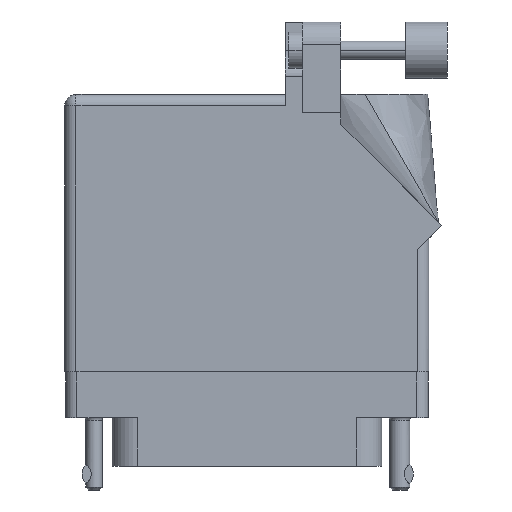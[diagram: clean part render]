
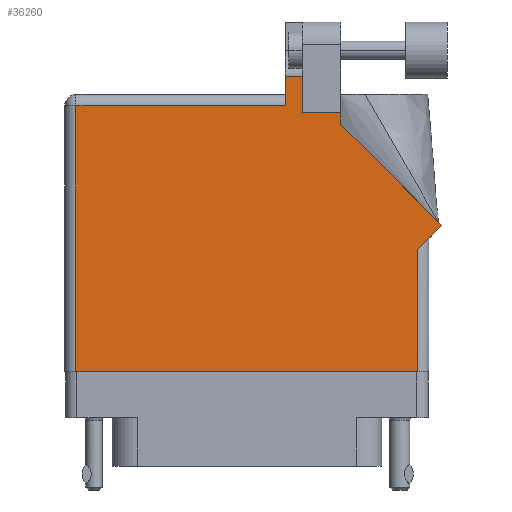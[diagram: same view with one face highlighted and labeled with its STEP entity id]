
A CAD part, front view. The second image highlights one B-rep face of the part: STEP entity #36260.
In plain terms, the highlighted face is planar.
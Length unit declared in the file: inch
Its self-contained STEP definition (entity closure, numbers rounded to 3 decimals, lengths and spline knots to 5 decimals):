
#535 = LINE ( 'NONE', #37012, #33537 ) ;
#968 = DIRECTION ( 'NONE',  ( -1., 0., 0. ) ) ;
#1126 = CARTESIAN_POINT ( 'NONE',  ( 1.005, 0.637, 0.455 ) ) ;
#1348 = CARTESIAN_POINT ( 'NONE',  ( 0.212, 1.368, 0.455 ) ) ;
#2317 = DIRECTION ( 'NONE',  ( 0., 1., 0. ) ) ;
#2615 = DIRECTION ( 'NONE',  ( 0., -1., 0. ) ) ;
#2785 = VECTOR ( 'NONE', #2317, 39.37008 ) ;
#3223 = LINE ( 'NONE', #24088, #43509 ) ;
#3614 = ORIENTED_EDGE ( 'NONE', *, *, #7888, .T. ) ;
#3955 = CARTESIAN_POINT ( 'NONE',  ( 0.306, 1.33, 0.455 ) ) ;
#5259 = EDGE_CURVE ( 'NONE', #46035, #9260, #48475, .T. ) ;
#5517 = EDGE_CURVE ( 'NONE', #9260, #12201, #16547, .T. ) ;
#5848 = VECTOR ( 'NONE', #28022, 39.37008 ) ;
#6562 = VECTOR ( 'NONE', #44307, 39.37008 ) ;
#7165 = ORIENTED_EDGE ( 'NONE', *, *, #14733, .T. ) ;
#7662 = VECTOR ( 'NONE', #46806, 39.37008 ) ;
#7813 = DIRECTION ( 'NONE',  ( 0., 1., 0. ) ) ;
#7818 = DIRECTION ( 'NONE',  ( -0.707, 0.707, 0. ) ) ;
#7888 = EDGE_CURVE ( 'NONE', #8590, #30130, #27279, .T. ) ;
#8525 = CARTESIAN_POINT ( 'NONE',  ( 0.519, 1.26442, 0.455 ) ) ;
#8590 = VERTEX_POINT ( 'NONE', #1348 ) ;
#8673 = VERTEX_POINT ( 'NONE', #17260 ) ;
#8853 = DIRECTION ( 'NONE',  ( 0., 0., -1. ) ) ;
#8906 = VECTOR ( 'NONE', #47312, 39.37008 ) ;
#9260 = VERTEX_POINT ( 'NONE', #21711 ) ;
#10191 = CARTESIAN_POINT ( 'NONE',  ( -0.943, -0.1, 0.455 ) ) ;
#10704 = ORIENTED_EDGE ( 'NONE', *, *, #5517, .T. ) ;
#11527 = AXIS2_PLACEMENT_3D ( 'NONE', #35538, #8853, #968 ) ;
#12143 = CARTESIAN_POINT ( 'NONE',  ( 0.212, 1.43, 0.455 ) ) ;
#12201 = VERTEX_POINT ( 'NONE', #40840 ) ;
#12972 = DIRECTION ( 'NONE',  ( -1., 0., 0. ) ) ;
#13647 = LINE ( 'NONE', #12143, #7662 ) ;
#14733 = EDGE_CURVE ( 'NONE', #47770, #28939, #3223, .T. ) ;
#15215 = CARTESIAN_POINT ( 'NONE',  ( -0.943, -0.1, 0.455 ) ) ;
#16235 = ORIENTED_EDGE ( 'NONE', *, *, #18946, .T. ) ;
#16547 = LINE ( 'NONE', #48149, #2785 ) ;
#17260 = CARTESIAN_POINT ( 'NONE',  ( 0.306, 1.5315, 0.455 ) ) ;
#17868 = CARTESIAN_POINT ( 'NONE',  ( 0.63677, 1.5315, 0.455 ) ) ;
#18648 = VERTEX_POINT ( 'NONE', #32779 ) ;
#18946 = EDGE_CURVE ( 'NONE', #26385, #8590, #13647, .T. ) ;
#20813 = ORIENTED_EDGE ( 'NONE', *, *, #5259, .T. ) ;
#20870 = EDGE_CURVE ( 'NONE', #30130, #46035, #36288, .T. ) ;
#21711 = CARTESIAN_POINT ( 'NONE',  ( 0.943, -0.1, 0.455 ) ) ;
#21772 = ORIENTED_EDGE ( 'NONE', *, *, #48228, .T. ) ;
#23064 = VECTOR ( 'NONE', #2615, 39.37008 ) ;
#23331 = VECTOR ( 'NONE', #7813, 39.37008 ) ;
#23992 = ORIENTED_EDGE ( 'NONE', *, *, #25083, .T. ) ;
#24088 = CARTESIAN_POINT ( 'NONE',  ( 0.519, 1.26442, 0.455 ) ) ;
#24949 = EDGE_CURVE ( 'NONE', #8673, #26385, #45022, .T. ) ;
#25083 = EDGE_CURVE ( 'NONE', #28939, #41791, #535, .T. ) ;
#26385 = VERTEX_POINT ( 'NONE', #49009 ) ;
#26912 = ORIENTED_EDGE ( 'NONE', *, *, #36675, .T. ) ;
#26986 = CARTESIAN_POINT ( 'NONE',  ( 0.306, 1.33, 0.455 ) ) ;
#27279 = LINE ( 'NONE', #35849, #46494 ) ;
#27842 = PLANE ( 'NONE',  #11527 ) ;
#28022 = DIRECTION ( 'NONE',  ( 1., 0., 0. ) ) ;
#28153 = DIRECTION ( 'NONE',  ( 0., 1., 0. ) ) ;
#28817 = CARTESIAN_POINT ( 'NONE',  ( 0.519, 1.33, 0.455 ) ) ;
#28939 = VERTEX_POINT ( 'NONE', #28817 ) ;
#29325 = ORIENTED_EDGE ( 'NONE', *, *, #24949, .T. ) ;
#29329 = CARTESIAN_POINT ( 'NONE',  ( -0.943, 1.368, 0.455 ) ) ;
#30130 = VERTEX_POINT ( 'NONE', #29329 ) ;
#31288 = ORIENTED_EDGE ( 'NONE', *, *, #20870, .T. ) ;
#32779 = CARTESIAN_POINT ( 'NONE',  ( 1.07571, 0.70771, 0.455 ) ) ;
#33537 = VECTOR ( 'NONE', #33597, 39.37008 ) ;
#33597 = DIRECTION ( 'NONE',  ( -1., 0., 0. ) ) ;
#35538 = CARTESIAN_POINT ( 'NONE',  ( -1.005, 1.43, 0.455 ) ) ;
#35849 = CARTESIAN_POINT ( 'NONE',  ( -1.005, 1.368, 0.455 ) ) ;
#36243 = EDGE_CURVE ( 'NONE', #12201, #18648, #47374, .T. ) ;
#36260 = ADVANCED_FACE ( 'NONE', ( #37156 ), #27842, .F. ) ;
#36288 = LINE ( 'NONE', #10191, #23064 ) ;
#36675 = EDGE_CURVE ( 'NONE', #18648, #47770, #40122, .T. ) ;
#37012 = CARTESIAN_POINT ( 'NONE',  ( 0.519, 1.33, 0.455 ) ) ;
#37086 = EDGE_LOOP ( 'NONE', ( #21772, #29325, #16235, #3614, #31288, #20813, #10704, #46174, #26912, #7165, #23992 ) ) ;
#37156 = FACE_OUTER_BOUND ( 'NONE', #37086, .T. ) ;
#38266 = VECTOR ( 'NONE', #7818, 39.37008 ) ;
#38532 = CARTESIAN_POINT ( 'NONE',  ( 1.07571, 0.70771, 0.455 ) ) ;
#39633 = CARTESIAN_POINT ( 'NONE',  ( -1.005, -0.1, 0.455 ) ) ;
#40122 = LINE ( 'NONE', #38532, #38266 ) ;
#40762 = LINE ( 'NONE', #3955, #23331 ) ;
#40840 = CARTESIAN_POINT ( 'NONE',  ( 0.943, 0.575, 0.455 ) ) ;
#41791 = VERTEX_POINT ( 'NONE', #26986 ) ;
#43509 = VECTOR ( 'NONE', #28153, 39.37008 ) ;
#44307 = DIRECTION ( 'NONE',  ( -1., 0., 0. ) ) ;
#45022 = LINE ( 'NONE', #17868, #6562 ) ;
#46035 = VERTEX_POINT ( 'NONE', #15215 ) ;
#46174 = ORIENTED_EDGE ( 'NONE', *, *, #36243, .T. ) ;
#46494 = VECTOR ( 'NONE', #12972, 39.37008 ) ;
#46806 = DIRECTION ( 'NONE',  ( 0., -1., 0. ) ) ;
#47312 = DIRECTION ( 'NONE',  ( 0.707, 0.707, 0. ) ) ;
#47374 = LINE ( 'NONE', #1126, #8906 ) ;
#47770 = VERTEX_POINT ( 'NONE', #8525 ) ;
#48149 = CARTESIAN_POINT ( 'NONE',  ( 0.943, 0.637, 0.455 ) ) ;
#48228 = EDGE_CURVE ( 'NONE', #41791, #8673, #40762, .T. ) ;
#48475 = LINE ( 'NONE', #39633, #5848 ) ;
#49009 = CARTESIAN_POINT ( 'NONE',  ( 0.212, 1.5315, 0.455 ) ) ;
